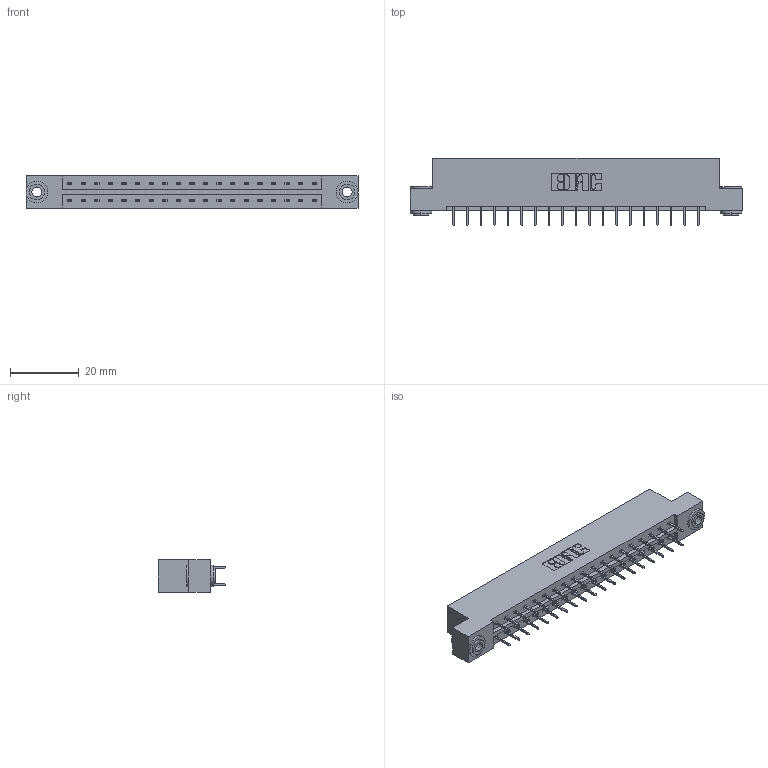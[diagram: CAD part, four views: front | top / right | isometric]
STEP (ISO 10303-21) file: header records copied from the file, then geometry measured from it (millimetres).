
FILE_DESCRIPTION (( 'STEP AP203' ), '1' );
FILE_NAME ('833-038-524-203.STEP', '2020-06-03T07:09:57', ( '' ), ( '' ), 'SwSTEP 2.0', 'SolidWorks 2020', '' );
FILE_SCHEMA (( 'CONFIG_CONTROL_DESIGN' ));
Length unit declared in the file: inch
Products named in the file (4): 345-250-002_345-250-002-102; 833 Part_Flush - .156 Dia - TH; 833-038-524-203; 345-292-001_345-293-124
Assembly tree (41 placements, depth 2):
  833-038-524-203
    833 Part_Flush - .156 Dia - TH
    345-292-001_345-293-124  x38
    345-250-002_345-250-002-102  x2
Bounding box: 96.82 x 19.69 x 9.4 mm (x, y, z)
Volume: 9632.1 mm3; surface area: 11188.6 mm2
Topology: 41 solids, 41 shells, 2280 faces, 6429 edges, 4130 vertices
Faces by surface type: plane 1676, cylinder 596, cone 8
Entity records: 15922 total; most frequent: CARTESIAN_POINT 2641, ORIENTED_EDGE 2570, DIRECTION 2331, EDGE_CURVE 1285, VECTOR 1137, LINE 1137, VERTEX_POINT 850, AXIS2_PLACEMENT_3D 597
